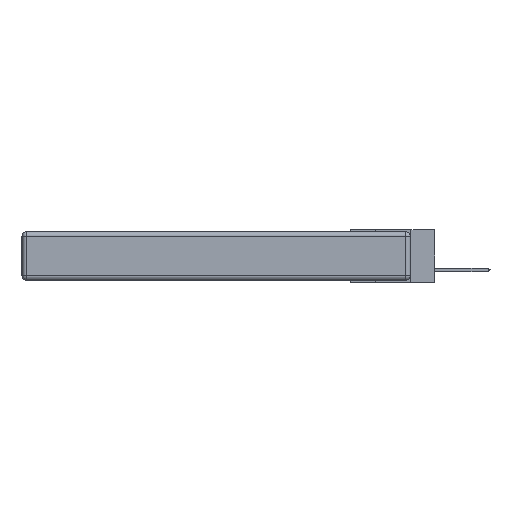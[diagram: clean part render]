
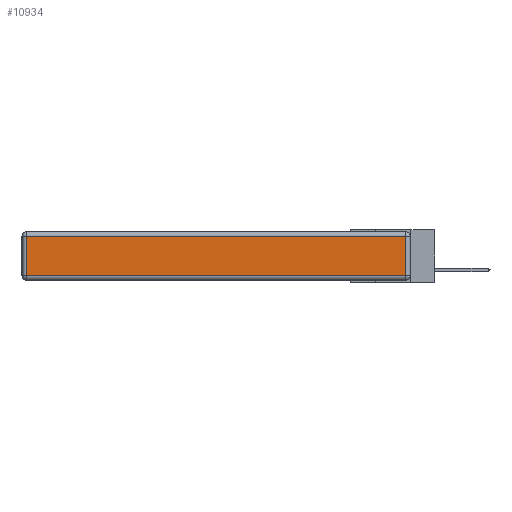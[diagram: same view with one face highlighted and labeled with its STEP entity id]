
A CAD part, left-side view. The second image highlights one B-rep face of the part: STEP entity #10934.
In plain terms, the highlighted planar face has unit normal (-1, 0, 0).
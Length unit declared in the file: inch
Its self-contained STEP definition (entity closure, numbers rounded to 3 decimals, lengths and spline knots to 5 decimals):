
#381 = EDGE_CURVE ( 'NONE', #8103, #21577, #12800, .T. ) ;
#454 = ORIENTED_EDGE ( 'NONE', *, *, #16655, .T. ) ;
#1088 = CARTESIAN_POINT ( 'NONE',  ( 0., 0.03, -0.03 ) ) ;
#1968 = EDGE_LOOP ( 'NONE', ( #24182, #20928, #22640, #454 ) ) ;
#2013 = LINE ( 'NONE', #12147, #16622 ) ;
#3112 = CARTESIAN_POINT ( 'NONE',  ( 0., 2.75, -0.03 ) ) ;
#3276 = DIRECTION ( 'NONE',  ( -1., 0., 0. ) ) ;
#5941 = EDGE_CURVE ( 'NONE', #14767, #8103, #18125, .T. ) ;
#8103 = VERTEX_POINT ( 'NONE', #9038 ) ;
#8918 = DIRECTION ( 'NONE',  ( 0., 0., 1. ) ) ;
#9038 = CARTESIAN_POINT ( 'NONE',  ( 0., 0.03, -0.313 ) ) ;
#9397 = DIRECTION ( 'NONE',  ( 0., 0., -1. ) ) ;
#9942 = VECTOR ( 'NONE', #20237, 39.37008 ) ;
#10934 = ADVANCED_FACE ( 'NONE', ( #26598 ), #15767, .T. ) ;
#12147 = CARTESIAN_POINT ( 'NONE',  ( 0., 2.72, -0.343 ) ) ;
#12800 = LINE ( 'NONE', #15538, #13629 ) ;
#13006 = VERTEX_POINT ( 'NONE', #31267 ) ;
#13629 = VECTOR ( 'NONE', #28508, 39.37008 ) ;
#14767 = VERTEX_POINT ( 'NONE', #24513 ) ;
#15538 = CARTESIAN_POINT ( 'NONE',  ( 0., 0.03, -0.343 ) ) ;
#15767 = PLANE ( 'NONE',  #31615 ) ;
#16622 = VECTOR ( 'NONE', #9397, 39.37008 ) ;
#16655 = EDGE_CURVE ( 'NONE', #13006, #14767, #2013, .T. ) ;
#18125 = LINE ( 'NONE', #20450, #9942 ) ;
#20237 = DIRECTION ( 'NONE',  ( 0., -1., 0. ) ) ;
#20450 = CARTESIAN_POINT ( 'NONE',  ( 0., 0., -0.313 ) ) ;
#20928 = ORIENTED_EDGE ( 'NONE', *, *, #381, .T. ) ;
#21577 = VERTEX_POINT ( 'NONE', #1088 ) ;
#22640 = ORIENTED_EDGE ( 'NONE', *, *, #26800, .T. ) ;
#24182 = ORIENTED_EDGE ( 'NONE', *, *, #5941, .T. ) ;
#24513 = CARTESIAN_POINT ( 'NONE',  ( 0., 2.72, -0.313 ) ) ;
#26018 = CARTESIAN_POINT ( 'NONE',  ( 0., 0., -0.343 ) ) ;
#26598 = FACE_OUTER_BOUND ( 'NONE', #1968, .T. ) ;
#26800 = EDGE_CURVE ( 'NONE', #21577, #13006, #27958, .T. ) ;
#27958 = LINE ( 'NONE', #3112, #33219 ) ;
#28508 = DIRECTION ( 'NONE',  ( 0., 0., 1. ) ) ;
#31267 = CARTESIAN_POINT ( 'NONE',  ( 0., 2.72, -0.03 ) ) ;
#31370 = DIRECTION ( 'NONE',  ( 0., 1., 0. ) ) ;
#31615 = AXIS2_PLACEMENT_3D ( 'NONE', #26018, #3276, #8918 ) ;
#33219 = VECTOR ( 'NONE', #31370, 39.37008 ) ;
